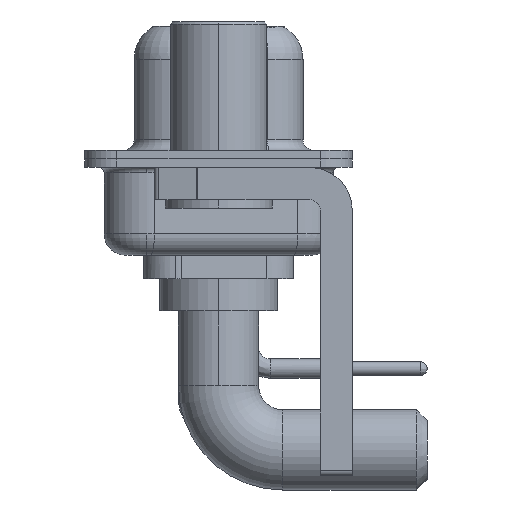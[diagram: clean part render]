
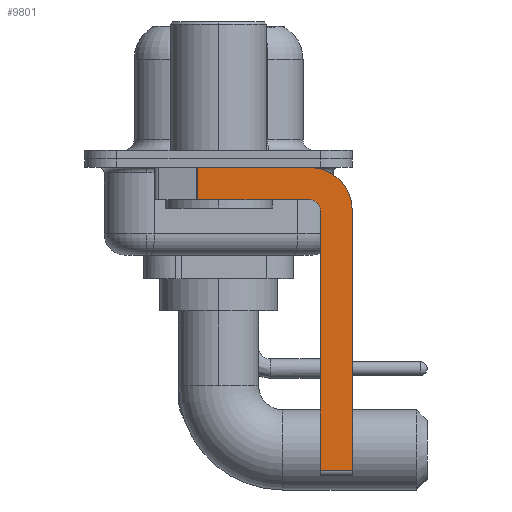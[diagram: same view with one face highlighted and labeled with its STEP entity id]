
A CAD part, left-side view. The second image highlights one B-rep face of the part: STEP entity #9801.
In plain terms, the highlighted planar face has unit normal (-1, 0, 0).
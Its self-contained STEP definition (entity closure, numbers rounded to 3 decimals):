
#671 = CARTESIAN_POINT ( 'NONE',  ( -2.9, -4.25, -2.4 ) ) ;
#791 = PLANE ( 'NONE',  #16933 ) ;
#815 = DIRECTION ( 'NONE',  ( 0., 0., -1. ) ) ;
#926 = CARTESIAN_POINT ( 'NONE',  ( -2.9, -6.25, -2.4 ) ) ;
#1000 = VECTOR ( 'NONE', #815, 1000. ) ;
#1061 = EDGE_CURVE ( 'NONE', #2125, #14960, #18257, .T. ) ;
#1892 = ORIENTED_EDGE ( 'NONE', *, *, #17101, .F. ) ;
#2125 = VERTEX_POINT ( 'NONE', #11705 ) ;
#2543 = DIRECTION ( 'NONE',  ( 0., 0., -1. ) ) ;
#2558 = CARTESIAN_POINT ( 'NONE',  ( -2.9, 3., -0.4 ) ) ;
#2662 = LINE ( 'NONE', #16686, #1000 ) ;
#3627 = VECTOR ( 'NONE', #11853, 1000. ) ;
#3889 = VERTEX_POINT ( 'NONE', #9112 ) ;
#3945 = CARTESIAN_POINT ( 'NONE',  ( -2.9, -4.25, -2.4 ) ) ;
#4022 = EDGE_CURVE ( 'NONE', #22131, #18320, #2662, .T. ) ;
#5472 = EDGE_CURVE ( 'NONE', #10718, #8240, #21638, .T. ) ;
#6011 = EDGE_CURVE ( 'NONE', #14960, #18320, #11622, .T. ) ;
#6965 = VECTOR ( 'NONE', #19927, 1000. ) ;
#7531 = ORIENTED_EDGE ( 'NONE', *, *, #9350, .F. ) ;
#7536 = DIRECTION ( 'NONE',  ( -1., 0., 0. ) ) ;
#7560 = DIRECTION ( 'NONE',  ( 0., 0., -1. ) ) ;
#8240 = VERTEX_POINT ( 'NONE', #13959 ) ;
#8377 = EDGE_CURVE ( 'NONE', #3889, #12437, #19592, .T. ) ;
#8608 = EDGE_CURVE ( 'NONE', #22131, #10718, #18859, .T. ) ;
#9112 = CARTESIAN_POINT ( 'NONE',  ( -2.9, -4.75, -14.55 ) ) ;
#9350 = EDGE_CURVE ( 'NONE', #8240, #12437, #13121, .T. ) ;
#9801 = ADVANCED_FACE ( 'NONE', ( #20238 ), #791, .F. ) ;
#10213 = DIRECTION ( 'NONE',  ( 0., -1., 0. ) ) ;
#10718 = VERTEX_POINT ( 'NONE', #16379 ) ;
#11186 = DIRECTION ( 'NONE',  ( 0., 0., -1. ) ) ;
#11622 = LINE ( 'NONE', #18653, #3627 ) ;
#11705 = CARTESIAN_POINT ( 'NONE',  ( -2.9, -4.75, -2.4 ) ) ;
#11853 = DIRECTION ( 'NONE',  ( 0., 1., 0. ) ) ;
#11883 = ORIENTED_EDGE ( 'NONE', *, *, #8608, .F. ) ;
#12437 = VERTEX_POINT ( 'NONE', #19733 ) ;
#12873 = VECTOR ( 'NONE', #2543, 1000. ) ;
#12914 = ORIENTED_EDGE ( 'NONE', *, *, #4022, .T. ) ;
#13121 = LINE ( 'NONE', #926, #12873 ) ;
#13959 = CARTESIAN_POINT ( 'NONE',  ( -2.9, -6.25, -2.4 ) ) ;
#14003 = CARTESIAN_POINT ( 'NONE',  ( -2.9, -4.75, -14.8 ) ) ;
#14688 = CARTESIAN_POINT ( 'NONE',  ( -2.9, -4.25, -2.4 ) ) ;
#14707 = VECTOR ( 'NONE', #10213, 1000. ) ;
#14960 = VERTEX_POINT ( 'NONE', #15522 ) ;
#15009 = AXIS2_PLACEMENT_3D ( 'NONE', #3945, #17987, #11186 ) ;
#15510 = CARTESIAN_POINT ( 'NONE',  ( -2.9, 0.978, -1.9 ) ) ;
#15522 = CARTESIAN_POINT ( 'NONE',  ( -2.9, -4.25, -1.9 ) ) ;
#16040 = VECTOR ( 'NONE', #22649, 1000. ) ;
#16379 = CARTESIAN_POINT ( 'NONE',  ( -2.9, -4.25, -0.4 ) ) ;
#16686 = CARTESIAN_POINT ( 'NONE',  ( -2.9, 0.978, -1.9 ) ) ;
#16795 = AXIS2_PLACEMENT_3D ( 'NONE', #14688, #7536, #19748 ) ;
#16933 = AXIS2_PLACEMENT_3D ( 'NONE', #671, #21748, #7560 ) ;
#17058 = ORIENTED_EDGE ( 'NONE', *, *, #6011, .F. ) ;
#17101 = EDGE_CURVE ( 'NONE', #3889, #2125, #19523, .T. ) ;
#17987 = DIRECTION ( 'NONE',  ( 1., 0., 0. ) ) ;
#18257 = CIRCLE ( 'NONE', #16795, 0.5 ) ;
#18320 = VERTEX_POINT ( 'NONE', #15510 ) ;
#18437 = CARTESIAN_POINT ( 'NONE',  ( -2.9, 0.978, -0.4 ) ) ;
#18653 = CARTESIAN_POINT ( 'NONE',  ( -2.9, -4.25, -1.9 ) ) ;
#18859 = LINE ( 'NONE', #2558, #14707 ) ;
#19523 = LINE ( 'NONE', #14003, #16040 ) ;
#19592 = LINE ( 'NONE', #21336, #6965 ) ;
#19733 = CARTESIAN_POINT ( 'NONE',  ( -2.9, -6.25, -14.55 ) ) ;
#19748 = DIRECTION ( 'NONE',  ( 0., 0., 1. ) ) ;
#19927 = DIRECTION ( 'NONE',  ( 0., -1., 0. ) ) ;
#20238 = FACE_OUTER_BOUND ( 'NONE', #21987, .T. ) ;
#21336 = CARTESIAN_POINT ( 'NONE',  ( -2.9, -4.25, -14.55 ) ) ;
#21638 = CIRCLE ( 'NONE', #15009, 2. ) ;
#21745 = ORIENTED_EDGE ( 'NONE', *, *, #8377, .T. ) ;
#21748 = DIRECTION ( 'NONE',  ( 1., 0., 0. ) ) ;
#21987 = EDGE_LOOP ( 'NONE', ( #11883, #12914, #17058, #22039, #1892, #21745, #7531, #22290 ) ) ;
#22039 = ORIENTED_EDGE ( 'NONE', *, *, #1061, .F. ) ;
#22131 = VERTEX_POINT ( 'NONE', #18437 ) ;
#22290 = ORIENTED_EDGE ( 'NONE', *, *, #5472, .F. ) ;
#22649 = DIRECTION ( 'NONE',  ( 0., 0., 1. ) ) ;
